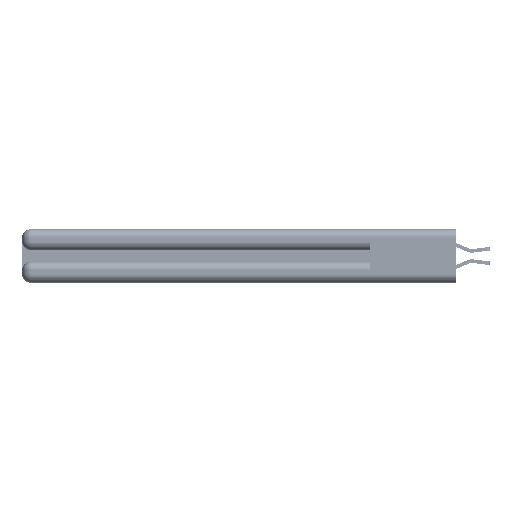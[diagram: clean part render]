
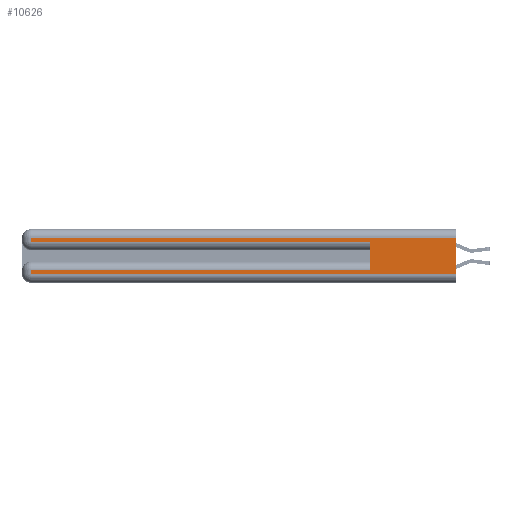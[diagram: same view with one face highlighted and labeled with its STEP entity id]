
A CAD part, left-side view. The second image highlights one B-rep face of the part: STEP entity #10626.
In plain terms, the highlighted planar face has unit normal (-1, 0, 0).
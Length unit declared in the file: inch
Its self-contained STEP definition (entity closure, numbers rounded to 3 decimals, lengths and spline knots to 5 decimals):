
#307 = ORIENTED_EDGE ( 'NONE', *, *, #39288, .F. ) ;
#384 = CARTESIAN_POINT ( 'NONE',  ( 0., 2.94, 0.06 ) ) ;
#698 = DIRECTION ( 'NONE',  ( 0., -1., 0. ) ) ;
#707 = DIRECTION ( 'NONE',  ( 0., 1., 0. ) ) ;
#1997 = DIRECTION ( 'NONE',  ( 0., 0., -1. ) ) ;
#2015 = VERTEX_POINT ( 'NONE', #39215 ) ;
#4332 = EDGE_CURVE ( 'NONE', #24238, #30076, #31859, .T. ) ;
#6249 = CARTESIAN_POINT ( 'NONE',  ( 0., 0., 0.06 ) ) ;
#7397 = LINE ( 'NONE', #32045, #43686 ) ;
#8275 = ORIENTED_EDGE ( 'NONE', *, *, #38527, .T. ) ;
#8394 = LINE ( 'NONE', #24203, #46438 ) ;
#9682 = LINE ( 'NONE', #17235, #26928 ) ;
#10188 = EDGE_CURVE ( 'NONE', #12201, #32382, #14941, .T. ) ;
#10300 = FACE_OUTER_BOUND ( 'NONE', #14553, .T. ) ;
#10626 = ADVANCED_FACE ( 'NONE', ( #10300 ), #16401, .F. ) ;
#10703 = DIRECTION ( 'NONE',  ( 1., 0., 0. ) ) ;
#10712 = CARTESIAN_POINT ( 'NONE',  ( 0., 0., 0.37 ) ) ;
#11455 = LINE ( 'NONE', #28782, #16124 ) ;
#12139 = VECTOR ( 'NONE', #698, 39.37008 ) ;
#12201 = VERTEX_POINT ( 'NONE', #17284 ) ;
#12275 = CARTESIAN_POINT ( 'NONE',  ( 0., 2.94, 0.31 ) ) ;
#12791 = CARTESIAN_POINT ( 'NONE',  ( 0., 2.94, 0.085 ) ) ;
#13157 = DIRECTION ( 'NONE',  ( 0., 0., -1. ) ) ;
#14553 = EDGE_LOOP ( 'NONE', ( #307, #8275, #46310, #29456, #22849, #26788, #46722, #45138 ) ) ;
#14941 = LINE ( 'NONE', #34179, #23584 ) ;
#15707 = CARTESIAN_POINT ( 'NONE',  ( 0., 0., 0.06 ) ) ;
#15780 = DIRECTION ( 'NONE',  ( 0., 1., 0. ) ) ;
#16124 = VECTOR ( 'NONE', #47427, 39.37008 ) ;
#16401 = PLANE ( 'NONE',  #26295 ) ;
#17235 = CARTESIAN_POINT ( 'NONE',  ( 0., 0., 0.285 ) ) ;
#17284 = CARTESIAN_POINT ( 'NONE',  ( 0., 0.6, 0.085 ) ) ;
#17722 = LINE ( 'NONE', #30324, #37799 ) ;
#18300 = VECTOR ( 'NONE', #39237, 39.37008 ) ;
#21041 = CARTESIAN_POINT ( 'NONE',  ( 0., 0.6, 0.285 ) ) ;
#21656 = CARTESIAN_POINT ( 'NONE',  ( 0., 0., 0.31 ) ) ;
#22849 = ORIENTED_EDGE ( 'NONE', *, *, #45550, .F. ) ;
#23584 = VECTOR ( 'NONE', #15780, 39.37008 ) ;
#24203 = CARTESIAN_POINT ( 'NONE',  ( 0., 0., 0.37 ) ) ;
#24238 = VERTEX_POINT ( 'NONE', #384 ) ;
#24434 = EDGE_CURVE ( 'NONE', #32382, #24238, #7397, .T. ) ;
#26295 = AXIS2_PLACEMENT_3D ( 'NONE', #10712, #10703, #33281 ) ;
#26788 = ORIENTED_EDGE ( 'NONE', *, *, #10188, .T. ) ;
#26928 = VECTOR ( 'NONE', #38790, 39.37008 ) ;
#28782 = CARTESIAN_POINT ( 'NONE',  ( 0., 0.6, 0.145 ) ) ;
#29456 = ORIENTED_EDGE ( 'NONE', *, *, #37415, .T. ) ;
#30076 = VERTEX_POINT ( 'NONE', #6249 ) ;
#30324 = CARTESIAN_POINT ( 'NONE',  ( 0., 0., 0.31 ) ) ;
#31859 = LINE ( 'NONE', #15707, #12139 ) ;
#32045 = CARTESIAN_POINT ( 'NONE',  ( 0., 2.94, 0.37 ) ) ;
#32382 = VERTEX_POINT ( 'NONE', #12791 ) ;
#32520 = VERTEX_POINT ( 'NONE', #21041 ) ;
#33281 = DIRECTION ( 'NONE',  ( 0., 0., -1. ) ) ;
#34179 = CARTESIAN_POINT ( 'NONE',  ( 0., 0., 0.085 ) ) ;
#35427 = CARTESIAN_POINT ( 'NONE',  ( 0., 2.94, 0.37 ) ) ;
#37415 = EDGE_CURVE ( 'NONE', #2015, #32520, #9682, .T. ) ;
#37799 = VECTOR ( 'NONE', #707, 39.37008 ) ;
#38527 = EDGE_CURVE ( 'NONE', #44419, #40985, #17722, .T. ) ;
#38790 = DIRECTION ( 'NONE',  ( 0., -1., 0. ) ) ;
#39215 = CARTESIAN_POINT ( 'NONE',  ( 0., 2.94, 0.285 ) ) ;
#39237 = DIRECTION ( 'NONE',  ( 0., 0., -1. ) ) ;
#39288 = EDGE_CURVE ( 'NONE', #44419, #30076, #8394, .T. ) ;
#40515 = EDGE_CURVE ( 'NONE', #40985, #2015, #46523, .T. ) ;
#40985 = VERTEX_POINT ( 'NONE', #12275 ) ;
#43686 = VECTOR ( 'NONE', #13157, 39.37008 ) ;
#44419 = VERTEX_POINT ( 'NONE', #21656 ) ;
#45138 = ORIENTED_EDGE ( 'NONE', *, *, #4332, .T. ) ;
#45550 = EDGE_CURVE ( 'NONE', #12201, #32520, #11455, .T. ) ;
#46310 = ORIENTED_EDGE ( 'NONE', *, *, #40515, .T. ) ;
#46438 = VECTOR ( 'NONE', #1997, 39.37008 ) ;
#46523 = LINE ( 'NONE', #35427, #18300 ) ;
#46722 = ORIENTED_EDGE ( 'NONE', *, *, #24434, .T. ) ;
#47427 = DIRECTION ( 'NONE',  ( 0., 0., 1. ) ) ;
